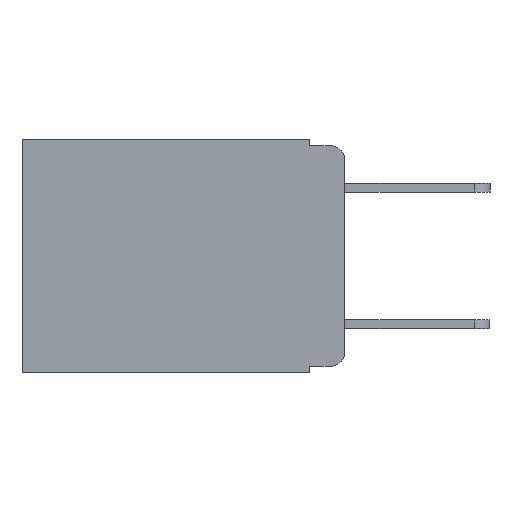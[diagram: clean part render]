
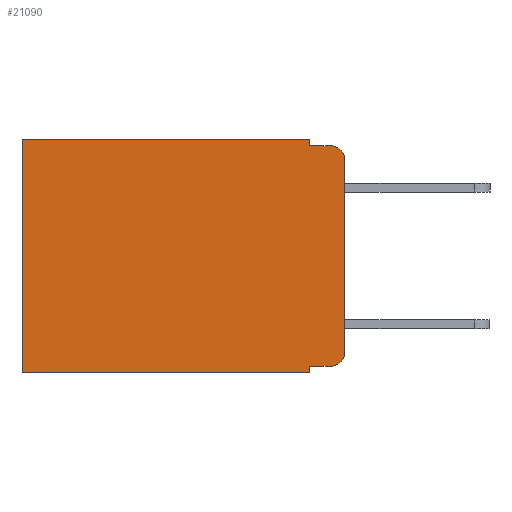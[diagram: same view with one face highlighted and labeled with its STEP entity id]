
A CAD part, left-side view. The second image highlights one B-rep face of the part: STEP entity #21090.
In plain terms, the highlighted planar face has unit normal (-1, 0, 0).
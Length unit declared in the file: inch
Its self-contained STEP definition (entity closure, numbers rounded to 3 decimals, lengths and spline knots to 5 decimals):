
#52 = VERTEX_POINT ( 'NONE', #19969 ) ;
#573 = DIRECTION ( 'NONE',  ( 1., 0., 0. ) ) ;
#609 = EDGE_CURVE ( 'NONE', #21485, #13987, #10095, .T. ) ;
#679 = CARTESIAN_POINT ( 'NONE',  ( 0.298, 0., -0.343 ) ) ;
#796 = CARTESIAN_POINT ( 'NONE',  ( 0.298, 0.473, 0. ) ) ;
#885 = LINE ( 'NONE', #9792, #5170 ) ;
#1136 = EDGE_CURVE ( 'NONE', #52, #15293, #13632, .T. ) ;
#1198 = CARTESIAN_POINT ( 'NONE',  ( 0.298, 0.051, -0.333 ) ) ;
#1495 = VERTEX_POINT ( 'NONE', #3864 ) ;
#1500 = ORIENTED_EDGE ( 'NONE', *, *, #20751, .F. ) ;
#1788 = DIRECTION ( 'NONE',  ( 0., 1., 0. ) ) ;
#2065 = ORIENTED_EDGE ( 'NONE', *, *, #1136, .T. ) ;
#2215 = DIRECTION ( 'NONE',  ( -1., 0., 0. ) ) ;
#2466 = DIRECTION ( 'NONE',  ( 0., 0., -1. ) ) ;
#2677 = EDGE_CURVE ( 'NONE', #11109, #15144, #14180, .T. ) ;
#2696 = CARTESIAN_POINT ( 'NONE',  ( 0.298, 0.02, -0.01 ) ) ;
#3136 = EDGE_CURVE ( 'NONE', #20962, #15293, #10055, .T. ) ;
#3507 = ORIENTED_EDGE ( 'NONE', *, *, #16164, .T. ) ;
#3864 = CARTESIAN_POINT ( 'NONE',  ( 0.298, 0., -0.313 ) ) ;
#3923 = EDGE_CURVE ( 'NONE', #15144, #1495, #13313, .T. ) ;
#3996 = CARTESIAN_POINT ( 'NONE',  ( 0.298, 0.02, -0.03 ) ) ;
#4098 = DIRECTION ( 'NONE',  ( -1., 0., 0. ) ) ;
#4340 = VECTOR ( 'NONE', #2466, 39.37008 ) ;
#4545 = DIRECTION ( 'NONE',  ( 0., 0., -1. ) ) ;
#5170 = VECTOR ( 'NONE', #4545, 39.37008 ) ;
#5389 = VERTEX_POINT ( 'NONE', #796 ) ;
#5458 = EDGE_LOOP ( 'NONE', ( #16466, #2065, #9914, #13748, #16740, #3507, #13725, #1500, #13467, #20225 ) ) ;
#5517 = EDGE_CURVE ( 'NONE', #16131, #5389, #14606, .T. ) ;
#5592 = CARTESIAN_POINT ( 'NONE',  ( 0.298, 0.051, -0.01 ) ) ;
#6343 = AXIS2_PLACEMENT_3D ( 'NONE', #3996, #4098, #15165 ) ;
#7056 = CARTESIAN_POINT ( 'NONE',  ( 0.298, 0.051, -0.343 ) ) ;
#8616 = CARTESIAN_POINT ( 'NONE',  ( 0.298, 0.051, 0. ) ) ;
#8624 = CARTESIAN_POINT ( 'NONE',  ( 0.298, 0.473, 0. ) ) ;
#8853 = VECTOR ( 'NONE', #11728, 39.37008 ) ;
#9117 = EDGE_CURVE ( 'NONE', #16131, #20962, #885, .T. ) ;
#9194 = LINE ( 'NONE', #8624, #22508 ) ;
#9792 = CARTESIAN_POINT ( 'NONE',  ( 0.298, 0.051, 0. ) ) ;
#9914 = ORIENTED_EDGE ( 'NONE', *, *, #3136, .F. ) ;
#10055 = LINE ( 'NONE', #17335, #14162 ) ;
#10095 = LINE ( 'NONE', #679, #14200 ) ;
#10306 = CARTESIAN_POINT ( 'NONE',  ( 0.298, 0.051, 0. ) ) ;
#10798 = CARTESIAN_POINT ( 'NONE',  ( 0.298, 0.02, -0.333 ) ) ;
#10970 = AXIS2_PLACEMENT_3D ( 'NONE', #12869, #2215, #14630 ) ;
#11109 = VERTEX_POINT ( 'NONE', #1198 ) ;
#11728 = DIRECTION ( 'NONE',  ( 0., 1., 0. ) ) ;
#12145 = DIRECTION ( 'NONE',  ( 0., 0., -1. ) ) ;
#12869 = CARTESIAN_POINT ( 'NONE',  ( 0.298, 0.02, -0.313 ) ) ;
#12890 = DIRECTION ( 'NONE',  ( 0., -1., 0. ) ) ;
#13057 = DIRECTION ( 'NONE',  ( 0., 0., -1. ) ) ;
#13313 = CIRCLE ( 'NONE', #10970, 0.02 ) ;
#13467 = ORIENTED_EDGE ( 'NONE', *, *, #2677, .T. ) ;
#13632 = CIRCLE ( 'NONE', #6343, 0.02 ) ;
#13725 = ORIENTED_EDGE ( 'NONE', *, *, #609, .F. ) ;
#13732 = FACE_OUTER_BOUND ( 'NONE', #5458, .T. ) ;
#13748 = ORIENTED_EDGE ( 'NONE', *, *, #9117, .F. ) ;
#13964 = DIRECTION ( 'NONE',  ( 0., 0., -1. ) ) ;
#13987 = VERTEX_POINT ( 'NONE', #16198 ) ;
#14162 = VECTOR ( 'NONE', #17254, 39.37008 ) ;
#14180 = LINE ( 'NONE', #15358, #18264 ) ;
#14200 = VECTOR ( 'NONE', #1788, 39.37008 ) ;
#14606 = LINE ( 'NONE', #20443, #8853 ) ;
#14630 = DIRECTION ( 'NONE',  ( 0., 0., -1. ) ) ;
#14883 = CARTESIAN_POINT ( 'NONE',  ( 0.298, 0., 0. ) ) ;
#15144 = VERTEX_POINT ( 'NONE', #10798 ) ;
#15165 = DIRECTION ( 'NONE',  ( 0., 0., -1. ) ) ;
#15293 = VERTEX_POINT ( 'NONE', #2696 ) ;
#15358 = CARTESIAN_POINT ( 'NONE',  ( 0.298, 0.051, -0.333 ) ) ;
#15668 = VECTOR ( 'NONE', #13964, 39.37008 ) ;
#16131 = VERTEX_POINT ( 'NONE', #10306 ) ;
#16164 = EDGE_CURVE ( 'NONE', #5389, #13987, #9194, .T. ) ;
#16198 = CARTESIAN_POINT ( 'NONE',  ( 0.298, 0.473, -0.343 ) ) ;
#16466 = ORIENTED_EDGE ( 'NONE', *, *, #19286, .F. ) ;
#16740 = ORIENTED_EDGE ( 'NONE', *, *, #5517, .T. ) ;
#16745 = LINE ( 'NONE', #8616, #15668 ) ;
#17254 = DIRECTION ( 'NONE',  ( 0., -1., 0. ) ) ;
#17335 = CARTESIAN_POINT ( 'NONE',  ( 0.298, 0.051, -0.01 ) ) ;
#17981 = AXIS2_PLACEMENT_3D ( 'NONE', #21673, #573, #13057 ) ;
#18264 = VECTOR ( 'NONE', #12890, 39.37008 ) ;
#18324 = LINE ( 'NONE', #14883, #4340 ) ;
#19286 = EDGE_CURVE ( 'NONE', #52, #1495, #18324, .T. ) ;
#19949 = PLANE ( 'NONE',  #17981 ) ;
#19969 = CARTESIAN_POINT ( 'NONE',  ( 0.298, 0., -0.03 ) ) ;
#20225 = ORIENTED_EDGE ( 'NONE', *, *, #3923, .T. ) ;
#20443 = CARTESIAN_POINT ( 'NONE',  ( 0.298, 0., 0. ) ) ;
#20751 = EDGE_CURVE ( 'NONE', #11109, #21485, #16745, .T. ) ;
#20962 = VERTEX_POINT ( 'NONE', #5592 ) ;
#21090 = ADVANCED_FACE ( 'NONE', ( #13732 ), #19949, .F. ) ;
#21485 = VERTEX_POINT ( 'NONE', #7056 ) ;
#21673 = CARTESIAN_POINT ( 'NONE',  ( 0.298, 0., 0. ) ) ;
#22508 = VECTOR ( 'NONE', #12145, 39.37008 ) ;
